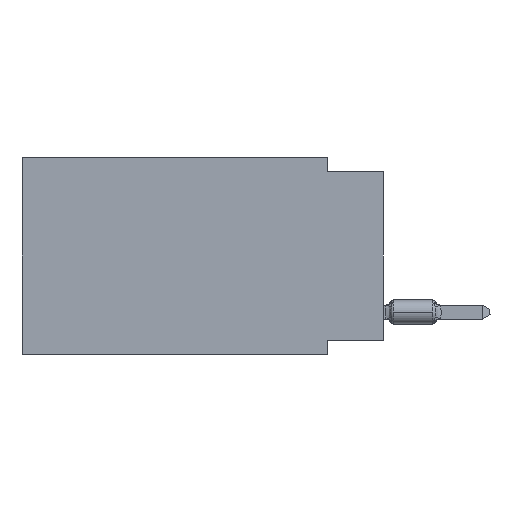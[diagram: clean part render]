
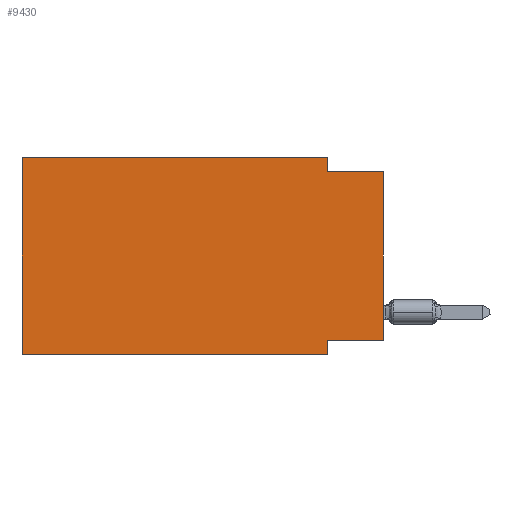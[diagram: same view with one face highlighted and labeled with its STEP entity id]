
A CAD part, left-side view. The second image highlights one B-rep face of the part: STEP entity #9430.
In plain terms, the highlighted planar face has unit normal (-1, 0, 0).
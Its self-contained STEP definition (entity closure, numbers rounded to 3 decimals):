
#804 = ORIENTED_EDGE ( 'NONE', *, *, #23295, .F. ) ;
#1988 = ORIENTED_EDGE ( 'NONE', *, *, #7546, .F. ) ;
#2132 = LINE ( 'NONE', #61524, #2616 ) ;
#2554 = DIRECTION ( 'NONE',  ( 0., -1., 0. ) ) ;
#2616 = VECTOR ( 'NONE', #82008, 1000. ) ;
#4038 = CARTESIAN_POINT ( 'NONE',  ( 0., 2.54, -0.635 ) ) ;
#5066 = LINE ( 'NONE', #38390, #45068 ) ;
#6155 = EDGE_CURVE ( 'NONE', #43902, #17167, #2132, .T. ) ;
#7546 = EDGE_CURVE ( 'NONE', #18299, #55876, #5066, .T. ) ;
#8503 = ORIENTED_EDGE ( 'NONE', *, *, #42262, .F. ) ;
#9430 = ADVANCED_FACE ( 'NONE', ( #70097 ), #44040, .F. ) ;
#11270 = CARTESIAN_POINT ( 'NONE',  ( 0., 2.54, -8.89 ) ) ;
#11551 = CARTESIAN_POINT ( 'NONE',  ( 0., 16.383, 0. ) ) ;
#13155 = DIRECTION ( 'NONE',  ( 0., -1., 0. ) ) ;
#14992 = ORIENTED_EDGE ( 'NONE', *, *, #59420, .T. ) ;
#15442 = VECTOR ( 'NONE', #43520, 1000. ) ;
#15750 = CARTESIAN_POINT ( 'NONE',  ( 0., 0., -0.635 ) ) ;
#16200 = VECTOR ( 'NONE', #70625, 1000. ) ;
#17157 = ORIENTED_EDGE ( 'NONE', *, *, #47254, .F. ) ;
#17167 = VERTEX_POINT ( 'NONE', #18672 ) ;
#18090 = LINE ( 'NONE', #11270, #31063 ) ;
#18299 = VERTEX_POINT ( 'NONE', #61922 ) ;
#18672 = CARTESIAN_POINT ( 'NONE',  ( 0., 2.54, -8.255 ) ) ;
#20244 = CARTESIAN_POINT ( 'NONE',  ( 0., 0., -8.255 ) ) ;
#22170 = LINE ( 'NONE', #67081, #37390 ) ;
#22441 = VECTOR ( 'NONE', #13155, 1000. ) ;
#22596 = VERTEX_POINT ( 'NONE', #27235 ) ;
#23295 = EDGE_CURVE ( 'NONE', #26634, #38321, #64260, .T. ) ;
#24358 = DIRECTION ( 'NONE',  ( 1., 0., 0. ) ) ;
#26391 = AXIS2_PLACEMENT_3D ( 'NONE', #11551, #24358, #37621 ) ;
#26399 = LINE ( 'NONE', #72130, #22441 ) ;
#26634 = VERTEX_POINT ( 'NONE', #31058 ) ;
#27235 = CARTESIAN_POINT ( 'NONE',  ( 0., 0., -0.635 ) ) ;
#31058 = CARTESIAN_POINT ( 'NONE',  ( 0., 2.54, 0. ) ) ;
#31063 = VECTOR ( 'NONE', #42513, 1000. ) ;
#36892 = CARTESIAN_POINT ( 'NONE',  ( 0., 16.383, 0. ) ) ;
#37390 = VECTOR ( 'NONE', #2554, 1000. ) ;
#37621 = DIRECTION ( 'NONE',  ( 0., 0., -1. ) ) ;
#38321 = VERTEX_POINT ( 'NONE', #4038 ) ;
#38390 = CARTESIAN_POINT ( 'NONE',  ( 0., 16.383, 0. ) ) ;
#42262 = EDGE_CURVE ( 'NONE', #38321, #22596, #42273, .T. ) ;
#42273 = LINE ( 'NONE', #15750, #15442 ) ;
#42513 = DIRECTION ( 'NONE',  ( 0., 0., -1. ) ) ;
#43304 = EDGE_CURVE ( 'NONE', #55876, #26634, #22170, .T. ) ;
#43520 = DIRECTION ( 'NONE',  ( 0., -1., 0. ) ) ;
#43902 = VERTEX_POINT ( 'NONE', #20244 ) ;
#44040 = PLANE ( 'NONE',  #26391 ) ;
#44384 = DIRECTION ( 'NONE',  ( 0., 0., 1. ) ) ;
#44590 = DIRECTION ( 'NONE',  ( 0., 0., -1. ) ) ;
#45002 = LINE ( 'NONE', #63801, #16200 ) ;
#45068 = VECTOR ( 'NONE', #44384, 1000. ) ;
#47254 = EDGE_CURVE ( 'NONE', #17167, #50471, #18090, .T. ) ;
#48807 = ORIENTED_EDGE ( 'NONE', *, *, #6155, .F. ) ;
#50471 = VERTEX_POINT ( 'NONE', #71692 ) ;
#52756 = EDGE_LOOP ( 'NONE', ( #64894, #8503, #804, #53422, #1988, #14992, #17157, #48807 ) ) ;
#53422 = ORIENTED_EDGE ( 'NONE', *, *, #43304, .F. ) ;
#55876 = VERTEX_POINT ( 'NONE', #36892 ) ;
#57552 = VECTOR ( 'NONE', #44590, 1000. ) ;
#59420 = EDGE_CURVE ( 'NONE', #18299, #50471, #26399, .T. ) ;
#61524 = CARTESIAN_POINT ( 'NONE',  ( 0., 0., -8.255 ) ) ;
#61922 = CARTESIAN_POINT ( 'NONE',  ( 0., 16.383, -8.89 ) ) ;
#63801 = CARTESIAN_POINT ( 'NONE',  ( 0., 0., 0. ) ) ;
#64260 = LINE ( 'NONE', #76651, #57552 ) ;
#64894 = ORIENTED_EDGE ( 'NONE', *, *, #83736, .T. ) ;
#67081 = CARTESIAN_POINT ( 'NONE',  ( 0., 16.383, 0. ) ) ;
#70097 = FACE_OUTER_BOUND ( 'NONE', #52756, .T. ) ;
#70625 = DIRECTION ( 'NONE',  ( 0., 0., 1. ) ) ;
#71692 = CARTESIAN_POINT ( 'NONE',  ( 0., 2.54, -8.89 ) ) ;
#72130 = CARTESIAN_POINT ( 'NONE',  ( 0., 16.383, -8.89 ) ) ;
#76651 = CARTESIAN_POINT ( 'NONE',  ( 0., 2.54, 0. ) ) ;
#82008 = DIRECTION ( 'NONE',  ( 0., 1., 0. ) ) ;
#83736 = EDGE_CURVE ( 'NONE', #43902, #22596, #45002, .T. ) ;
